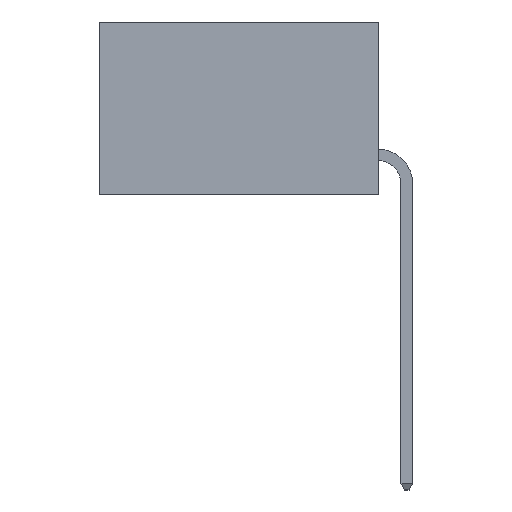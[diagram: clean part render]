
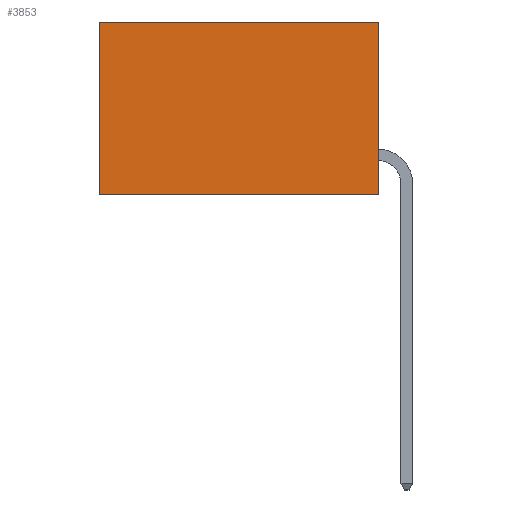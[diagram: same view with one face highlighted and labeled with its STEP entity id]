
A CAD part, left-side view. The second image highlights one B-rep face of the part: STEP entity #3853.
In plain terms, the highlighted planar face has unit normal (-1, 0, 0).
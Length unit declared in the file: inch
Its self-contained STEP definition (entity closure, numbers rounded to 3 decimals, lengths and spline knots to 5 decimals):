
#53 = LINE ( 'NONE', #12125, #14478 ) ;
#501 = VERTEX_POINT ( 'NONE', #10709 ) ;
#868 = EDGE_LOOP ( 'NONE', ( #17522, #4867, #14057, #10961 ) ) ;
#1024 = VECTOR ( 'NONE', #17780, 39.37008 ) ;
#1270 = DIRECTION ( 'NONE',  ( 0., 1., 0. ) ) ;
#1666 = EDGE_CURVE ( 'NONE', #12899, #2409, #12248, .T. ) ;
#1890 = CARTESIAN_POINT ( 'NONE',  ( 0.2615, 0., -0.37 ) ) ;
#2302 = LINE ( 'NONE', #13341, #3191 ) ;
#2409 = VERTEX_POINT ( 'NONE', #6727 ) ;
#3191 = VECTOR ( 'NONE', #13309, 39.37008 ) ;
#3853 = ADVANCED_FACE ( 'NONE', ( #7593 ), #16828, .F. ) ;
#4867 = ORIENTED_EDGE ( 'NONE', *, *, #10221, .F. ) ;
#6727 = CARTESIAN_POINT ( 'NONE',  ( 0.2615, 0., -0.37 ) ) ;
#7593 = FACE_OUTER_BOUND ( 'NONE', #868, .T. ) ;
#9126 = VERTEX_POINT ( 'NONE', #9553 ) ;
#9553 = CARTESIAN_POINT ( 'NONE',  ( 0.2615, 0.6, 0. ) ) ;
#9890 = CARTESIAN_POINT ( 'NONE',  ( 0.2615, 0., -0.37 ) ) ;
#10110 = LINE ( 'NONE', #1890, #13695 ) ;
#10221 = EDGE_CURVE ( 'NONE', #2409, #501, #10110, .T. ) ;
#10661 = CARTESIAN_POINT ( 'NONE',  ( 0.2615, 0., 0. ) ) ;
#10709 = CARTESIAN_POINT ( 'NONE',  ( 0.2615, 0.6, -0.37 ) ) ;
#10961 = ORIENTED_EDGE ( 'NONE', *, *, #11919, .T. ) ;
#11687 = DIRECTION ( 'NONE',  ( 0., 0., -1. ) ) ;
#11796 = DIRECTION ( 'NONE',  ( 1., 0., 0. ) ) ;
#11919 = EDGE_CURVE ( 'NONE', #12899, #9126, #53, .T. ) ;
#12013 = DIRECTION ( 'NONE',  ( 0., 1., 0. ) ) ;
#12125 = CARTESIAN_POINT ( 'NONE',  ( 0.2615, 0., 0. ) ) ;
#12248 = LINE ( 'NONE', #9890, #1024 ) ;
#12899 = VERTEX_POINT ( 'NONE', #10661 ) ;
#13309 = DIRECTION ( 'NONE',  ( 0., 0., -1. ) ) ;
#13341 = CARTESIAN_POINT ( 'NONE',  ( 0.2615, 0.6, -0.37 ) ) ;
#13695 = VECTOR ( 'NONE', #1270, 39.37008 ) ;
#14057 = ORIENTED_EDGE ( 'NONE', *, *, #1666, .F. ) ;
#14478 = VECTOR ( 'NONE', #12013, 39.37008 ) ;
#14831 = CARTESIAN_POINT ( 'NONE',  ( 0.2615, 0., -0.37 ) ) ;
#14892 = EDGE_CURVE ( 'NONE', #9126, #501, #2302, .T. ) ;
#15313 = AXIS2_PLACEMENT_3D ( 'NONE', #14831, #11796, #11687 ) ;
#16828 = PLANE ( 'NONE',  #15313 ) ;
#17522 = ORIENTED_EDGE ( 'NONE', *, *, #14892, .T. ) ;
#17780 = DIRECTION ( 'NONE',  ( 0., 0., -1. ) ) ;
